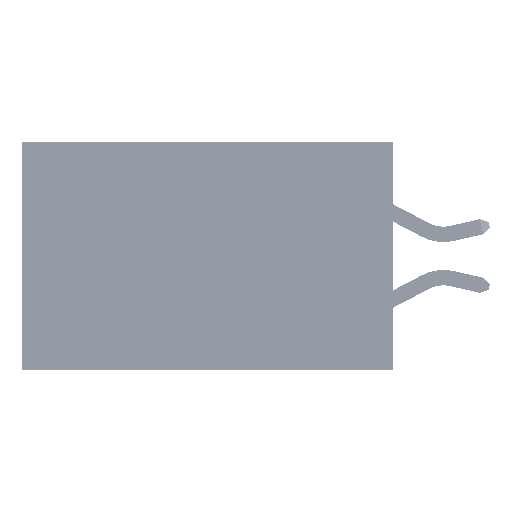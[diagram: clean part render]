
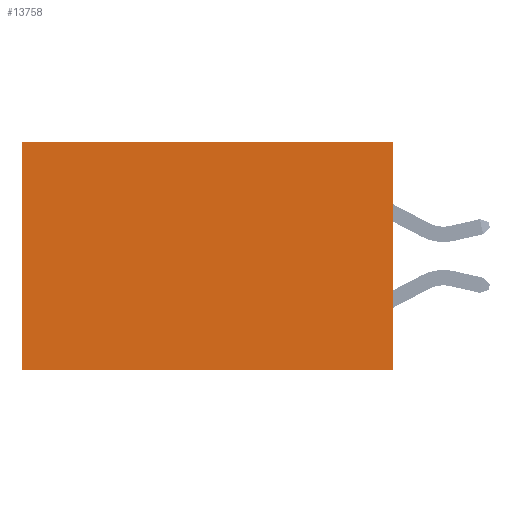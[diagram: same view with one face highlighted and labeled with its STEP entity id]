
A CAD part, left-side view. The second image highlights one B-rep face of the part: STEP entity #13758.
In plain terms, the highlighted planar face has unit normal (-1, 0, 0).
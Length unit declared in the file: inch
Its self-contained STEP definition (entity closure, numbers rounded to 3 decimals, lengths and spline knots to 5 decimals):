
#29 = DIRECTION ( 'NONE',  ( 0., 1., 0. ) ) ;
#1558 = CARTESIAN_POINT ( 'NONE',  ( 0.2875, 0., -0.37 ) ) ;
#3369 = LINE ( 'NONE', #43848, #9715 ) ;
#3786 = EDGE_CURVE ( 'NONE', #36935, #12576, #9215, .T. ) ;
#4126 = DIRECTION ( 'NONE',  ( 1., 0., 0. ) ) ;
#4620 = ORIENTED_EDGE ( 'NONE', *, *, #8583, .F. ) ;
#8583 = EDGE_CURVE ( 'NONE', #26420, #38189, #18590, .T. ) ;
#9215 = LINE ( 'NONE', #19049, #38133 ) ;
#9248 = EDGE_CURVE ( 'NONE', #38189, #12576, #33449, .T. ) ;
#9715 = VECTOR ( 'NONE', #29, 39.37008 ) ;
#12576 = VERTEX_POINT ( 'NONE', #32730 ) ;
#12881 = CARTESIAN_POINT ( 'NONE',  ( 0.2875, 0., -0.37 ) ) ;
#13466 = CARTESIAN_POINT ( 'NONE',  ( 0.2875, 0.6, 0. ) ) ;
#13758 = ADVANCED_FACE ( 'NONE', ( #36023 ), #47655, .F. ) ;
#18321 = ORIENTED_EDGE ( 'NONE', *, *, #40397, .T. ) ;
#18590 = LINE ( 'NONE', #19043, #26676 ) ;
#19043 = CARTESIAN_POINT ( 'NONE',  ( 0.2875, 0., 0. ) ) ;
#19049 = CARTESIAN_POINT ( 'NONE',  ( 0.2875, 0.6, 0. ) ) ;
#22921 = DIRECTION ( 'NONE',  ( 0., 0., -1. ) ) ;
#23196 = DIRECTION ( 'NONE',  ( 0., 1., 0. ) ) ;
#26420 = VERTEX_POINT ( 'NONE', #38688 ) ;
#26430 = DIRECTION ( 'NONE',  ( 0., 0., -1. ) ) ;
#26676 = VECTOR ( 'NONE', #30001, 39.37008 ) ;
#28115 = ORIENTED_EDGE ( 'NONE', *, *, #3786, .T. ) ;
#30001 = DIRECTION ( 'NONE',  ( 0., 0., -1. ) ) ;
#30063 = AXIS2_PLACEMENT_3D ( 'NONE', #37747, #4126, #26430 ) ;
#32730 = CARTESIAN_POINT ( 'NONE',  ( 0.2875, 0.6, -0.37 ) ) ;
#33449 = LINE ( 'NONE', #1558, #41577 ) ;
#34153 = EDGE_LOOP ( 'NONE', ( #28115, #47336, #4620, #18321 ) ) ;
#36023 = FACE_OUTER_BOUND ( 'NONE', #34153, .T. ) ;
#36935 = VERTEX_POINT ( 'NONE', #13466 ) ;
#37747 = CARTESIAN_POINT ( 'NONE',  ( 0.2875, 0., 0. ) ) ;
#38133 = VECTOR ( 'NONE', #22921, 39.37008 ) ;
#38189 = VERTEX_POINT ( 'NONE', #12881 ) ;
#38688 = CARTESIAN_POINT ( 'NONE',  ( 0.2875, 0., 0. ) ) ;
#40397 = EDGE_CURVE ( 'NONE', #26420, #36935, #3369, .T. ) ;
#41577 = VECTOR ( 'NONE', #23196, 39.37008 ) ;
#43848 = CARTESIAN_POINT ( 'NONE',  ( 0.2875, 0., 0. ) ) ;
#47336 = ORIENTED_EDGE ( 'NONE', *, *, #9248, .F. ) ;
#47655 = PLANE ( 'NONE',  #30063 ) ;
